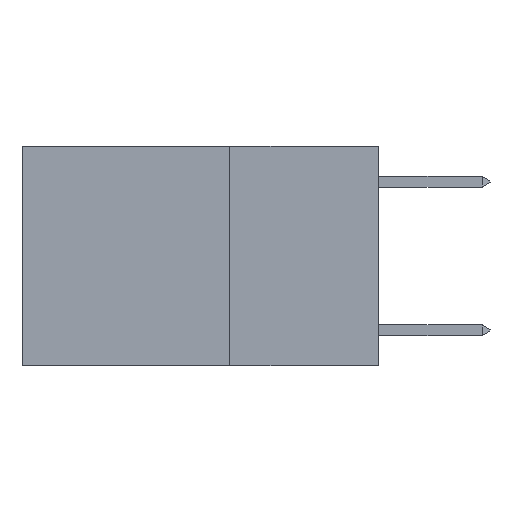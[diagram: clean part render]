
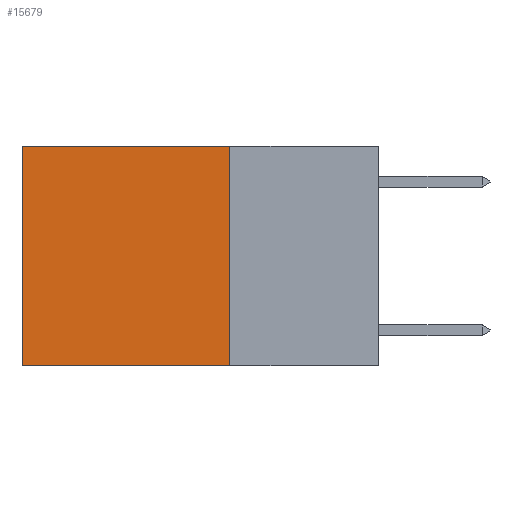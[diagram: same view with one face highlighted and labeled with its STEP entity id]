
A CAD part, left-side view. The second image highlights one B-rep face of the part: STEP entity #15679.
In plain terms, the highlighted planar face has unit normal (-1, 0, 0).
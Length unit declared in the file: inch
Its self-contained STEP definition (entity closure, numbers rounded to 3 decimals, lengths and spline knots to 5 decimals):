
#891 = VECTOR ( 'NONE', #13111, 39.37008 ) ;
#1722 = EDGE_CURVE ( 'NONE', #10705, #20714, #15316, .T. ) ;
#2926 = CARTESIAN_POINT ( 'NONE',  ( 0.2625, 0.25, -0.37 ) ) ;
#3626 = VERTEX_POINT ( 'NONE', #11942 ) ;
#3970 = DIRECTION ( 'NONE',  ( 1., 0., 0. ) ) ;
#4210 = VECTOR ( 'NONE', #6831, 39.37008 ) ;
#5695 = EDGE_CURVE ( 'NONE', #10705, #11836, #5752, .T. ) ;
#5752 = LINE ( 'NONE', #14217, #19027 ) ;
#5963 = CARTESIAN_POINT ( 'NONE',  ( 0.2625, 0.25, 0. ) ) ;
#6131 = CARTESIAN_POINT ( 'NONE',  ( 0.2625, 0.25, -0.37 ) ) ;
#6376 = CARTESIAN_POINT ( 'NONE',  ( 0.2625, 0.25, 0. ) ) ;
#6831 = DIRECTION ( 'NONE',  ( 0., 0., -1. ) ) ;
#6873 = ORIENTED_EDGE ( 'NONE', *, *, #12399, .T. ) ;
#7094 = ORIENTED_EDGE ( 'NONE', *, *, #1722, .F. ) ;
#7503 = AXIS2_PLACEMENT_3D ( 'NONE', #5963, #3970, #12672 ) ;
#10705 = VERTEX_POINT ( 'NONE', #13829 ) ;
#11096 = PLANE ( 'NONE',  #7503 ) ;
#11554 = EDGE_LOOP ( 'NONE', ( #6873, #17174, #7094, #21040 ) ) ;
#11828 = VECTOR ( 'NONE', #13315, 39.37008 ) ;
#11836 = VERTEX_POINT ( 'NONE', #13085 ) ;
#11942 = CARTESIAN_POINT ( 'NONE',  ( 0.2625, 0.6, -0.37 ) ) ;
#12399 = EDGE_CURVE ( 'NONE', #11836, #3626, #15221, .T. ) ;
#12561 = FACE_OUTER_BOUND ( 'NONE', #11554, .T. ) ;
#12672 = DIRECTION ( 'NONE',  ( 0., 0., -1. ) ) ;
#12909 = DIRECTION ( 'NONE',  ( 0., 1., 0. ) ) ;
#13085 = CARTESIAN_POINT ( 'NONE',  ( 0.2625, 0.6, 0. ) ) ;
#13111 = DIRECTION ( 'NONE',  ( 0., 0., -1. ) ) ;
#13315 = DIRECTION ( 'NONE',  ( 0., 1., 0. ) ) ;
#13829 = CARTESIAN_POINT ( 'NONE',  ( 0.2625, 0.25, 0. ) ) ;
#14217 = CARTESIAN_POINT ( 'NONE',  ( 0.2625, 0.25, 0. ) ) ;
#15221 = LINE ( 'NONE', #20465, #4210 ) ;
#15316 = LINE ( 'NONE', #6376, #891 ) ;
#15679 = ADVANCED_FACE ( 'NONE', ( #12561 ), #11096, .F. ) ;
#16236 = EDGE_CURVE ( 'NONE', #20714, #3626, #18192, .T. ) ;
#17174 = ORIENTED_EDGE ( 'NONE', *, *, #16236, .F. ) ;
#18192 = LINE ( 'NONE', #2926, #11828 ) ;
#19027 = VECTOR ( 'NONE', #12909, 39.37008 ) ;
#20465 = CARTESIAN_POINT ( 'NONE',  ( 0.2625, 0.6, 0. ) ) ;
#20714 = VERTEX_POINT ( 'NONE', #6131 ) ;
#21040 = ORIENTED_EDGE ( 'NONE', *, *, #5695, .T. ) ;
